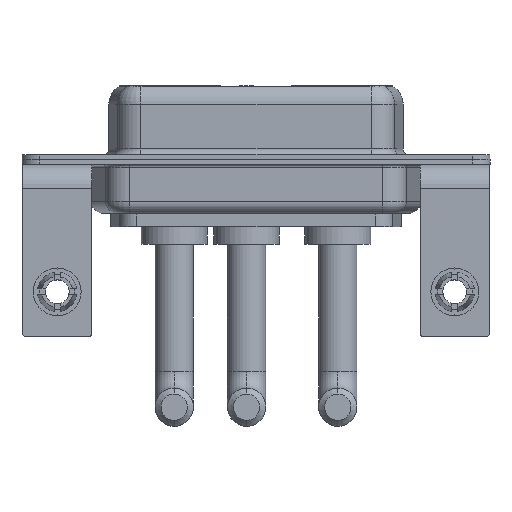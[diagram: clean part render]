
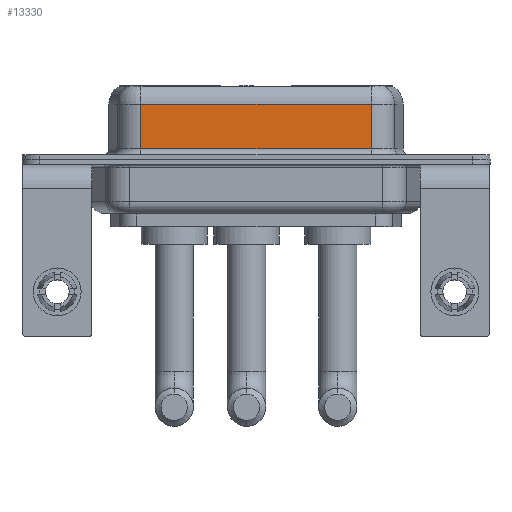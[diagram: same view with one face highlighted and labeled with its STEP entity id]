
A CAD part, front view. The second image highlights one B-rep face of the part: STEP entity #13330.
In plain terms, the highlighted planar face has unit normal (0, -1, 0).
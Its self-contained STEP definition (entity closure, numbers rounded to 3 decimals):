
#235 = PLANE ( 'NONE',  #9076 ) ;
#320 = ORIENTED_EDGE ( 'NONE', *, *, #8271, .T. ) ;
#460 = CARTESIAN_POINT ( 'NONE',  ( 26.287, -3.95, 4.65 ) ) ;
#514 = CARTESIAN_POINT ( 'NONE',  ( 26.287, -3.95, 6.4 ) ) ;
#848 = VERTEX_POINT ( 'NONE', #460 ) ;
#1146 = EDGE_CURVE ( 'NONE', #848, #14769, #11908, .T. ) ;
#1378 = CARTESIAN_POINT ( 'NONE',  ( 26.287, -3.95, 6.4 ) ) ;
#1384 = LINE ( 'NONE', #7811, #6256 ) ;
#1438 = EDGE_CURVE ( 'NONE', #12688, #2541, #1384, .T. ) ;
#1466 = DIRECTION ( 'NONE',  ( 0., 0., 1. ) ) ;
#2541 = VERTEX_POINT ( 'NONE', #12828 ) ;
#2647 = VECTOR ( 'NONE', #12652, 1000. ) ;
#2782 = DIRECTION ( 'NONE',  ( 0., 0., -1. ) ) ;
#4528 = ORIENTED_EDGE ( 'NONE', *, *, #1438, .T. ) ;
#4700 = CARTESIAN_POINT ( 'NONE',  ( 26.287, -3.95, 4.65 ) ) ;
#5253 = DIRECTION ( 'NONE',  ( 0., 1., 0. ) ) ;
#6256 = VECTOR ( 'NONE', #2782, 1000. ) ;
#6567 = VECTOR ( 'NONE', #9700, 1000. ) ;
#6741 = EDGE_LOOP ( 'NONE', ( #14641, #10483, #4528, #320 ) ) ;
#7316 = EDGE_CURVE ( 'NONE', #848, #12688, #13604, .T. ) ;
#7811 = CARTESIAN_POINT ( 'NONE',  ( 7.013, -3.95, 6.4 ) ) ;
#8271 = EDGE_CURVE ( 'NONE', #2541, #14769, #14098, .T. ) ;
#8868 = FACE_OUTER_BOUND ( 'NONE', #6741, .T. ) ;
#9076 = AXIS2_PLACEMENT_3D ( 'NONE', #1378, #5253, #1466 ) ;
#9700 = DIRECTION ( 'NONE',  ( -1., 0., 0. ) ) ;
#9899 = VECTOR ( 'NONE', #13055, 1000. ) ;
#10483 = ORIENTED_EDGE ( 'NONE', *, *, #7316, .T. ) ;
#11908 = LINE ( 'NONE', #514, #9899 ) ;
#12652 = DIRECTION ( 'NONE',  ( 1., 0., 0. ) ) ;
#12688 = VERTEX_POINT ( 'NONE', #14754 ) ;
#12828 = CARTESIAN_POINT ( 'NONE',  ( 7.013, -3.95, 0.9 ) ) ;
#13055 = DIRECTION ( 'NONE',  ( 0., 0., -1. ) ) ;
#13330 = ADVANCED_FACE ( 'NONE', ( #8868 ), #235, .F. ) ;
#13604 = LINE ( 'NONE', #4700, #6567 ) ;
#14084 = CARTESIAN_POINT ( 'NONE',  ( 26.287, -3.95, 0.9 ) ) ;
#14098 = LINE ( 'NONE', #15315, #2647 ) ;
#14641 = ORIENTED_EDGE ( 'NONE', *, *, #1146, .F. ) ;
#14754 = CARTESIAN_POINT ( 'NONE',  ( 7.013, -3.95, 4.65 ) ) ;
#14769 = VERTEX_POINT ( 'NONE', #14084 ) ;
#15315 = CARTESIAN_POINT ( 'NONE',  ( 26.287, -3.95, 0.9 ) ) ;
